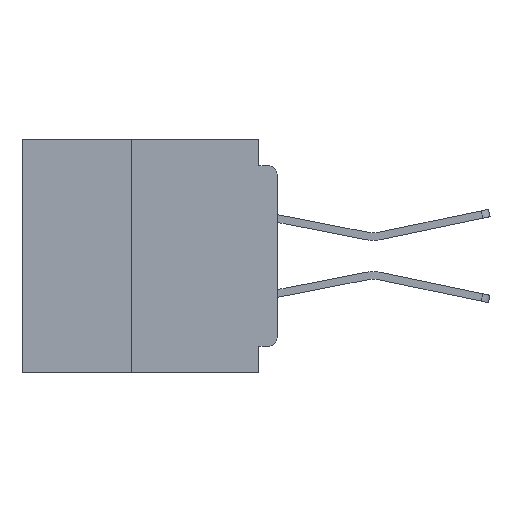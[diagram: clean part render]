
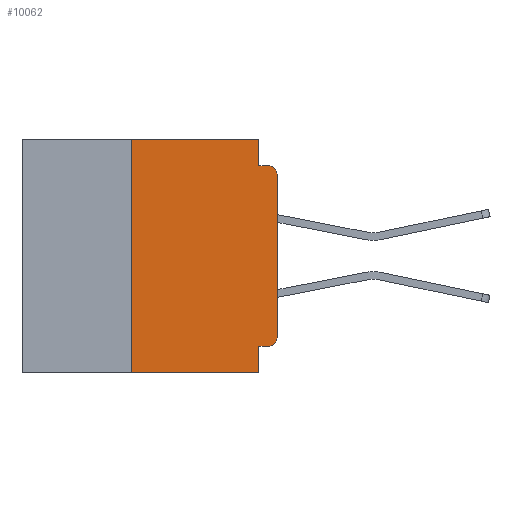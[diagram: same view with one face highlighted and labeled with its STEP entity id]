
A CAD part, left-side view. The second image highlights one B-rep face of the part: STEP entity #10062.
In plain terms, the highlighted planar face has unit normal (-1, 0, 0).
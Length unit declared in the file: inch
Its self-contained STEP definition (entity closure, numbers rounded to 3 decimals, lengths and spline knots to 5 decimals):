
#346 = DIRECTION ( 'NONE',  ( 0., -1., 0. ) ) ;
#1771 = CARTESIAN_POINT ( 'NONE',  ( 0., 0., 0. ) ) ;
#2097 = VECTOR ( 'NONE', #7113, 39.37008 ) ;
#2592 = VERTEX_POINT ( 'NONE', #3729 ) ;
#2891 = VECTOR ( 'NONE', #6321, 39.37008 ) ;
#3152 = ORIENTED_EDGE ( 'NONE', *, *, #6261, .T. ) ;
#3729 = CARTESIAN_POINT ( 'NONE',  ( 0., 0.25, 0. ) ) ;
#4304 = CARTESIAN_POINT ( 'NONE',  ( 0., 0.25, -0.4 ) ) ;
#5148 = LINE ( 'NONE', #54559, #26756 ) ;
#6261 = EDGE_CURVE ( 'NONE', #40189, #18082, #51669, .T. ) ;
#6321 = DIRECTION ( 'NONE',  ( 0., 0., 1. ) ) ;
#6530 = DIRECTION ( 'NONE',  ( -1., 0., 0. ) ) ;
#6826 = CIRCLE ( 'NONE', #55271, 0.015 ) ;
#7113 = DIRECTION ( 'NONE',  ( 0., -1., 0. ) ) ;
#7154 = CARTESIAN_POINT ( 'NONE',  ( 0., 0.031, -0.4 ) ) ;
#7682 = VERTEX_POINT ( 'NONE', #14051 ) ;
#8237 = DIRECTION ( 'NONE',  ( -1., 0., 0. ) ) ;
#8433 = VERTEX_POINT ( 'NONE', #15691 ) ;
#8691 = EDGE_CURVE ( 'NONE', #52256, #18082, #54463, .T. ) ;
#8734 = EDGE_CURVE ( 'NONE', #2592, #43894, #41780, .T. ) ;
#8775 = VECTOR ( 'NONE', #26017, 39.37008 ) ;
#10062 = ADVANCED_FACE ( 'NONE', ( #20145 ), #36308, .F. ) ;
#10789 = EDGE_CURVE ( 'NONE', #40189, #2592, #5148, .T. ) ;
#11956 = EDGE_CURVE ( 'NONE', #8433, #7682, #38734, .T. ) ;
#13047 = CARTESIAN_POINT ( 'NONE',  ( 0., 0., -0.34 ) ) ;
#13621 = LINE ( 'NONE', #24287, #2097 ) ;
#14051 = CARTESIAN_POINT ( 'NONE',  ( 0., 0.015, -0.045 ) ) ;
#14090 = AXIS2_PLACEMENT_3D ( 'NONE', #32349, #6530, #36691 ) ;
#14417 = LINE ( 'NONE', #1771, #2891 ) ;
#14859 = DIRECTION ( 'NONE',  ( 1., 0., 0. ) ) ;
#15691 = CARTESIAN_POINT ( 'NONE',  ( 0., 0., -0.06 ) ) ;
#15873 = VERTEX_POINT ( 'NONE', #13047 ) ;
#17675 = AXIS2_PLACEMENT_3D ( 'NONE', #19032, #14859, #44927 ) ;
#18082 = VERTEX_POINT ( 'NONE', #7154 ) ;
#18700 = CARTESIAN_POINT ( 'NONE',  ( 0., 0.031, -0.045 ) ) ;
#19032 = CARTESIAN_POINT ( 'NONE',  ( 0., 0.437, 0. ) ) ;
#19683 = DIRECTION ( 'NONE',  ( 0., 1., 0. ) ) ;
#20145 = FACE_OUTER_BOUND ( 'NONE', #27839, .T. ) ;
#20347 = EDGE_CURVE ( 'NONE', #44872, #52256, #41018, .T. ) ;
#22432 = CARTESIAN_POINT ( 'NONE',  ( 0., 0.031, 0. ) ) ;
#23455 = ORIENTED_EDGE ( 'NONE', *, *, #10789, .F. ) ;
#23794 = CARTESIAN_POINT ( 'NONE',  ( 0., 0., -0.355 ) ) ;
#24287 = CARTESIAN_POINT ( 'NONE',  ( 0., 0., -0.045 ) ) ;
#24586 = DIRECTION ( 'NONE',  ( 0., 0., 1. ) ) ;
#24733 = VERTEX_POINT ( 'NONE', #18700 ) ;
#24938 = EDGE_CURVE ( 'NONE', #24733, #7682, #13621, .T. ) ;
#26017 = DIRECTION ( 'NONE',  ( 0., 0., -1. ) ) ;
#26204 = CARTESIAN_POINT ( 'NONE',  ( 0., 0.437, 0. ) ) ;
#26756 = VECTOR ( 'NONE', #24586, 39.37008 ) ;
#27839 = EDGE_LOOP ( 'NONE', ( #44214, #45554, #36858, #40904, #30795, #23455, #3152, #45603, #35597, #49635 ) ) ;
#30251 = EDGE_CURVE ( 'NONE', #15873, #8433, #14417, .T. ) ;
#30795 = ORIENTED_EDGE ( 'NONE', *, *, #8734, .F. ) ;
#30863 = VECTOR ( 'NONE', #39898, 39.37008 ) ;
#32349 = CARTESIAN_POINT ( 'NONE',  ( 0., 0.015, -0.06 ) ) ;
#34023 = CARTESIAN_POINT ( 'NONE',  ( 0., 0.437, -0.4 ) ) ;
#34071 = CARTESIAN_POINT ( 'NONE',  ( 0., 0.015, -0.34 ) ) ;
#34657 = CARTESIAN_POINT ( 'NONE',  ( 0., 0.015, -0.355 ) ) ;
#35597 = ORIENTED_EDGE ( 'NONE', *, *, #20347, .F. ) ;
#35615 = CARTESIAN_POINT ( 'NONE',  ( 0., 0.031, 0. ) ) ;
#36308 = PLANE ( 'NONE',  #17675 ) ;
#36691 = DIRECTION ( 'NONE',  ( 0., 0., -1. ) ) ;
#36858 = ORIENTED_EDGE ( 'NONE', *, *, #24938, .F. ) ;
#38337 = DIRECTION ( 'NONE',  ( 0., -1., 0. ) ) ;
#38389 = DIRECTION ( 'NONE',  ( 0., 0., -1. ) ) ;
#38734 = CIRCLE ( 'NONE', #14090, 0.015 ) ;
#39898 = DIRECTION ( 'NONE',  ( 0., 0., -1. ) ) ;
#40189 = VERTEX_POINT ( 'NONE', #4304 ) ;
#40293 = VECTOR ( 'NONE', #38337, 39.37008 ) ;
#40436 = VECTOR ( 'NONE', #346, 39.37008 ) ;
#40904 = ORIENTED_EDGE ( 'NONE', *, *, #42032, .F. ) ;
#41018 = LINE ( 'NONE', #23794, #51054 ) ;
#41780 = LINE ( 'NONE', #26204, #40436 ) ;
#42032 = EDGE_CURVE ( 'NONE', #43894, #24733, #53650, .T. ) ;
#43894 = VERTEX_POINT ( 'NONE', #22432 ) ;
#44214 = ORIENTED_EDGE ( 'NONE', *, *, #30251, .T. ) ;
#44872 = VERTEX_POINT ( 'NONE', #34657 ) ;
#44927 = DIRECTION ( 'NONE',  ( 0., 0., -1. ) ) ;
#45324 = CARTESIAN_POINT ( 'NONE',  ( 0., 0.031, -0.355 ) ) ;
#45554 = ORIENTED_EDGE ( 'NONE', *, *, #11956, .T. ) ;
#45603 = ORIENTED_EDGE ( 'NONE', *, *, #8691, .F. ) ;
#47402 = CARTESIAN_POINT ( 'NONE',  ( 0., 0.031, -0.4 ) ) ;
#49635 = ORIENTED_EDGE ( 'NONE', *, *, #52497, .T. ) ;
#51054 = VECTOR ( 'NONE', #19683, 39.37008 ) ;
#51669 = LINE ( 'NONE', #34023, #40293 ) ;
#52256 = VERTEX_POINT ( 'NONE', #45324 ) ;
#52497 = EDGE_CURVE ( 'NONE', #44872, #15873, #6826, .T. ) ;
#53650 = LINE ( 'NONE', #35615, #30863 ) ;
#54463 = LINE ( 'NONE', #47402, #8775 ) ;
#54559 = CARTESIAN_POINT ( 'NONE',  ( 0., 0.25, -0.4 ) ) ;
#55271 = AXIS2_PLACEMENT_3D ( 'NONE', #34071, #8237, #38389 ) ;
